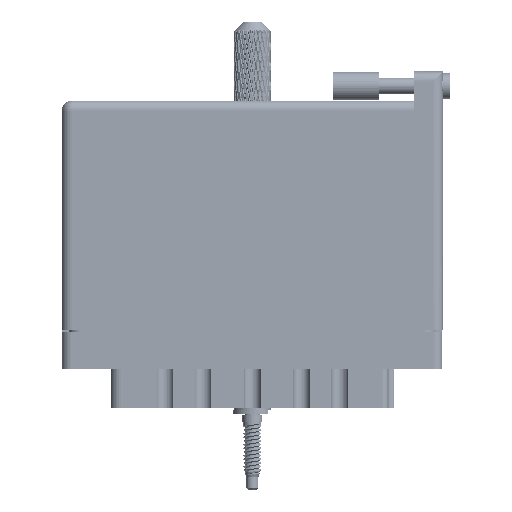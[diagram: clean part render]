
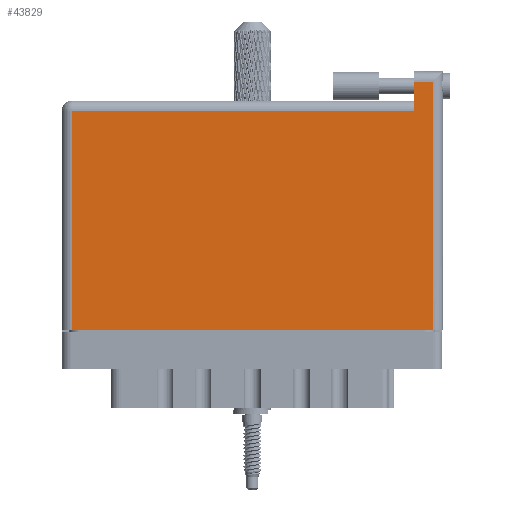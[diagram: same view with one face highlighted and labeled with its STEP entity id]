
A CAD part, front view. The second image highlights one B-rep face of the part: STEP entity #43829.
In plain terms, the highlighted face is planar.
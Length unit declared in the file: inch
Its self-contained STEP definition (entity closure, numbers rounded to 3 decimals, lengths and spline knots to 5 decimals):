
#6053 = CARTESIAN_POINT ( 'NONE',  ( 0.07, 1.496, 0. ) ) ;
#8084 = DIRECTION ( 'NONE',  ( -1., 0., 0. ) ) ;
#10146 = LINE ( 'NONE', #94915, #50532 ) ;
#11154 = PLANE ( 'NONE',  #22047 ) ;
#12423 = CARTESIAN_POINT ( 'NONE',  ( 2.403, 1.696, 0. ) ) ;
#12805 = LINE ( 'NONE', #114913, #34442 ) ;
#14399 = VECTOR ( 'NONE', #97147, 39.37008 ) ;
#16559 = EDGE_CURVE ( 'NONE', #99375, #63788, #10146, .T. ) ;
#16890 = DIRECTION ( 'NONE',  ( 0., -1., 0. ) ) ;
#20366 = DIRECTION ( 'NONE',  ( -1., 0., 0. ) ) ;
#21559 = DIRECTION ( 'NONE',  ( 0., 0., -1. ) ) ;
#22047 = AXIS2_PLACEMENT_3D ( 'NONE', #57879, #21559, #20366 ) ;
#30083 = ORIENTED_EDGE ( 'NONE', *, *, #55039, .T. ) ;
#34442 = VECTOR ( 'NONE', #51517, 39.37008 ) ;
#40006 = EDGE_CURVE ( 'NONE', #114708, #99375, #12805, .T. ) ;
#43829 = ADVANCED_FACE ( 'NONE', ( #58251 ), #11154, .F. ) ;
#50501 = CARTESIAN_POINT ( 'NONE',  ( 2.53, 1.766, 0. ) ) ;
#50532 = VECTOR ( 'NONE', #103286, 39.37008 ) ;
#51517 = DIRECTION ( 'NONE',  ( 0., -1., 0. ) ) ;
#55039 = EDGE_CURVE ( 'NONE', #91710, #114708, #83139, .T. ) ;
#57099 = VECTOR ( 'NONE', #66122, 39.37008 ) ;
#57879 = CARTESIAN_POINT ( 'NONE',  ( 0., 1.566, 0. ) ) ;
#57957 = VECTOR ( 'NONE', #16890, 39.37008 ) ;
#58251 = FACE_OUTER_BOUND ( 'NONE', #108218, .T. ) ;
#62353 = EDGE_CURVE ( 'NONE', #69659, #91710, #66664, .T. ) ;
#63322 = LINE ( 'NONE', #106997, #84907 ) ;
#63788 = VERTEX_POINT ( 'NONE', #101560 ) ;
#63891 = ORIENTED_EDGE ( 'NONE', *, *, #62353, .T. ) ;
#66122 = DIRECTION ( 'NONE',  ( -1., 0., 0. ) ) ;
#66664 = LINE ( 'NONE', #81750, #57957 ) ;
#69659 = VERTEX_POINT ( 'NONE', #12423 ) ;
#70100 = ORIENTED_EDGE ( 'NONE', *, *, #80516, .T. ) ;
#75107 = CARTESIAN_POINT ( 'NONE',  ( 2.403, 1.496, 0. ) ) ;
#75644 = EDGE_CURVE ( 'NONE', #63788, #76860, #106420, .T. ) ;
#76860 = VERTEX_POINT ( 'NONE', #114837 ) ;
#80516 = EDGE_CURVE ( 'NONE', #76860, #69659, #63322, .T. ) ;
#81237 = ORIENTED_EDGE ( 'NONE', *, *, #75644, .T. ) ;
#81750 = CARTESIAN_POINT ( 'NONE',  ( 2.403, 1.766, 0. ) ) ;
#83139 = LINE ( 'NONE', #102175, #57099 ) ;
#83561 = CARTESIAN_POINT ( 'NONE',  ( 0.07, 0., 0. ) ) ;
#84907 = VECTOR ( 'NONE', #8084, 39.37008 ) ;
#89853 = ORIENTED_EDGE ( 'NONE', *, *, #16559, .T. ) ;
#91710 = VERTEX_POINT ( 'NONE', #75107 ) ;
#94915 = CARTESIAN_POINT ( 'NONE',  ( 0., 0., 0. ) ) ;
#97147 = DIRECTION ( 'NONE',  ( 0., 1., 0. ) ) ;
#97652 = ORIENTED_EDGE ( 'NONE', *, *, #40006, .T. ) ;
#99375 = VERTEX_POINT ( 'NONE', #83561 ) ;
#101560 = CARTESIAN_POINT ( 'NONE',  ( 2.53, 0., 0. ) ) ;
#102175 = CARTESIAN_POINT ( 'NONE',  ( 0., 1.496, 0. ) ) ;
#103286 = DIRECTION ( 'NONE',  ( 1., 0., 0. ) ) ;
#106420 = LINE ( 'NONE', #50501, #14399 ) ;
#106997 = CARTESIAN_POINT ( 'NONE',  ( 0., 1.696, 0. ) ) ;
#108218 = EDGE_LOOP ( 'NONE', ( #89853, #81237, #70100, #63891, #30083, #97652 ) ) ;
#114708 = VERTEX_POINT ( 'NONE', #6053 ) ;
#114837 = CARTESIAN_POINT ( 'NONE',  ( 2.53, 1.696, 0. ) ) ;
#114913 = CARTESIAN_POINT ( 'NONE',  ( 0.07, 0., 0. ) ) ;
